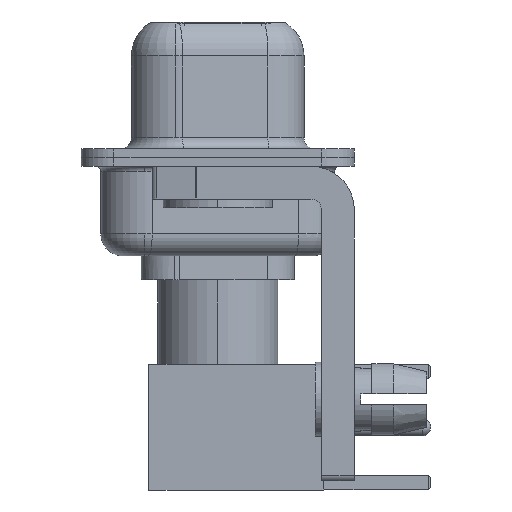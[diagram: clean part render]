
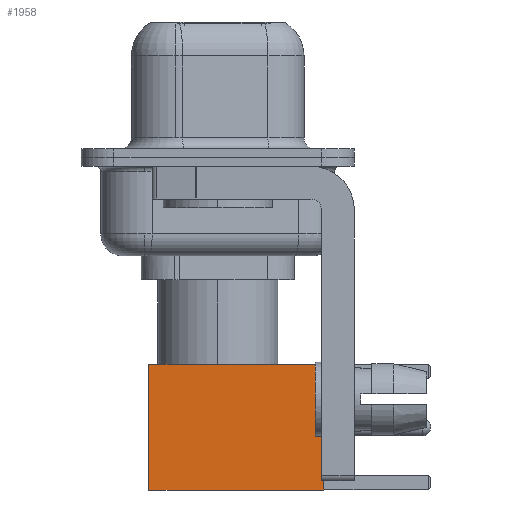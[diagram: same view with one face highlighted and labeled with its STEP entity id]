
A CAD part, left-side view. The second image highlights one B-rep face of the part: STEP entity #1958.
In plain terms, the highlighted face is planar.
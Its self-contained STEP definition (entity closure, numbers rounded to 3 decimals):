
#196 = CARTESIAN_POINT ( 'NONE',  ( 2.875, 2.875, 8. ) ) ;
#1019 = VERTEX_POINT ( 'NONE', #11750 ) ;
#1174 = CARTESIAN_POINT ( 'NONE',  ( 2.875, 2.875, 0. ) ) ;
#1382 = EDGE_LOOP ( 'NONE', ( #8965, #16876, #2748, #4710 ) ) ;
#1593 = DIRECTION ( 'NONE',  ( -1., 0., 0. ) ) ;
#1958 = ADVANCED_FACE ( 'NONE', ( #8918 ), #11615, .T. ) ;
#2634 = CARTESIAN_POINT ( 'NONE',  ( 0., 2.875, 8. ) ) ;
#2748 = ORIENTED_EDGE ( 'NONE', *, *, #13147, .F. ) ;
#3313 = VECTOR ( 'NONE', #1593, 1000. ) ;
#3365 = VERTEX_POINT ( 'NONE', #10069 ) ;
#3440 = DIRECTION ( 'NONE',  ( 0., 0., 1. ) ) ;
#4110 = AXIS2_PLACEMENT_3D ( 'NONE', #15683, #9437, #3440 ) ;
#4217 = EDGE_CURVE ( 'NONE', #4383, #4515, #5306, .T. ) ;
#4235 = LINE ( 'NONE', #9542, #3313 ) ;
#4383 = VERTEX_POINT ( 'NONE', #196 ) ;
#4515 = VERTEX_POINT ( 'NONE', #1174 ) ;
#4710 = ORIENTED_EDGE ( 'NONE', *, *, #6875, .F. ) ;
#5166 = EDGE_CURVE ( 'NONE', #4515, #1019, #4235, .T. ) ;
#5306 = LINE ( 'NONE', #10757, #16613 ) ;
#5770 = DIRECTION ( 'NONE',  ( -1., 0., 0. ) ) ;
#6145 = LINE ( 'NONE', #14409, #11618 ) ;
#6875 = EDGE_CURVE ( 'NONE', #4383, #3365, #16424, .T. ) ;
#8918 = FACE_OUTER_BOUND ( 'NONE', #1382, .T. ) ;
#8965 = ORIENTED_EDGE ( 'NONE', *, *, #4217, .T. ) ;
#9437 = DIRECTION ( 'NONE',  ( 0., 1., 0. ) ) ;
#9542 = CARTESIAN_POINT ( 'NONE',  ( 0., 2.875, 0. ) ) ;
#10069 = CARTESIAN_POINT ( 'NONE',  ( -2.875, 2.875, 8. ) ) ;
#10757 = CARTESIAN_POINT ( 'NONE',  ( 2.875, 2.875, 0. ) ) ;
#10851 = DIRECTION ( 'NONE',  ( 0., 0., -1. ) ) ;
#11615 = PLANE ( 'NONE',  #4110 ) ;
#11618 = VECTOR ( 'NONE', #16705, 1000. ) ;
#11750 = CARTESIAN_POINT ( 'NONE',  ( -2.875, 2.875, 0. ) ) ;
#12283 = VECTOR ( 'NONE', #5770, 1000. ) ;
#13147 = EDGE_CURVE ( 'NONE', #3365, #1019, #6145, .T. ) ;
#14409 = CARTESIAN_POINT ( 'NONE',  ( -2.875, 2.875, 0. ) ) ;
#15683 = CARTESIAN_POINT ( 'NONE',  ( 2.875, 2.875, 0. ) ) ;
#16424 = LINE ( 'NONE', #2634, #12283 ) ;
#16613 = VECTOR ( 'NONE', #10851, 1000. ) ;
#16705 = DIRECTION ( 'NONE',  ( 0., 0., -1. ) ) ;
#16876 = ORIENTED_EDGE ( 'NONE', *, *, #5166, .T. ) ;
